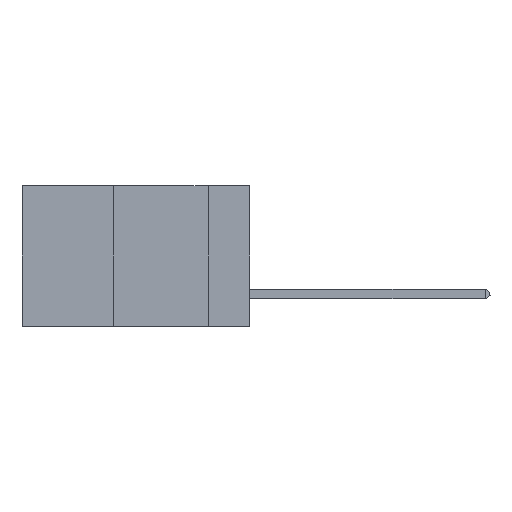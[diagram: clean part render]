
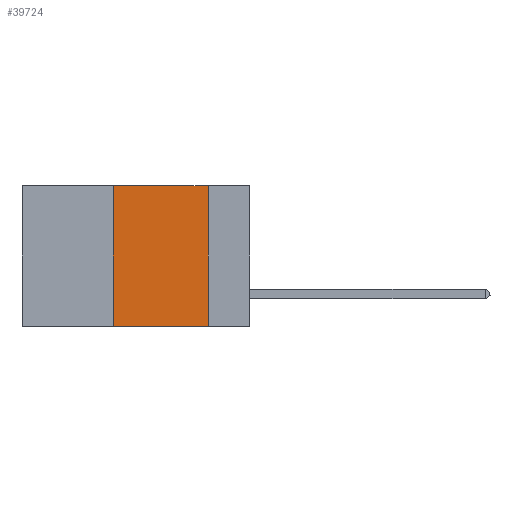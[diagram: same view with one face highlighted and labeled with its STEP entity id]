
A CAD part, left-side view. The second image highlights one B-rep face of the part: STEP entity #39724.
In plain terms, the highlighted planar face has unit normal (-1, 0, 0).
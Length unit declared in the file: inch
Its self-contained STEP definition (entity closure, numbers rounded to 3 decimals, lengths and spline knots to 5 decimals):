
#577 = FACE_OUTER_BOUND ( 'NONE', #27280, .T. ) ;
#1694 = DIRECTION ( 'NONE',  ( 0., 0., 1. ) ) ;
#2815 = VERTEX_POINT ( 'NONE', #20544 ) ;
#5615 = CARTESIAN_POINT ( 'NONE',  ( 0., 0.36, 0. ) ) ;
#7092 = CARTESIAN_POINT ( 'NONE',  ( 0., 0.11, 0. ) ) ;
#7485 = VECTOR ( 'NONE', #1694, 39.37008 ) ;
#9587 = ORIENTED_EDGE ( 'NONE', *, *, #45591, .F. ) ;
#9704 = DIRECTION ( 'NONE',  ( 0., -1., 0. ) ) ;
#9716 = VECTOR ( 'NONE', #43113, 39.37008 ) ;
#10158 = AXIS2_PLACEMENT_3D ( 'NONE', #39242, #46768, #35796 ) ;
#10191 = CARTESIAN_POINT ( 'NONE',  ( 0., 0.36, -0.37 ) ) ;
#10508 = VECTOR ( 'NONE', #29801, 39.37008 ) ;
#10557 = VERTEX_POINT ( 'NONE', #10191 ) ;
#14171 = ORIENTED_EDGE ( 'NONE', *, *, #23688, .T. ) ;
#16242 = VERTEX_POINT ( 'NONE', #26214 ) ;
#17302 = EDGE_CURVE ( 'NONE', #16242, #23471, #37473, .T. ) ;
#20544 = CARTESIAN_POINT ( 'NONE',  ( 0., 0.36, 0. ) ) ;
#20882 = PLANE ( 'NONE',  #10158 ) ;
#21519 = LINE ( 'NONE', #5615, #7485 ) ;
#22015 = LINE ( 'NONE', #35717, #34338 ) ;
#23471 = VERTEX_POINT ( 'NONE', #38985 ) ;
#23688 = EDGE_CURVE ( 'NONE', #10557, #23471, #22015, .T. ) ;
#26214 = CARTESIAN_POINT ( 'NONE',  ( 0., 0.11, 0. ) ) ;
#27280 = EDGE_LOOP ( 'NONE', ( #32638, #46162, #9587, #14171 ) ) ;
#29801 = DIRECTION ( 'NONE',  ( 0., 0., -1. ) ) ;
#31628 = CARTESIAN_POINT ( 'NONE',  ( 0., 0.6, 0. ) ) ;
#32638 = ORIENTED_EDGE ( 'NONE', *, *, #17302, .F. ) ;
#34338 = VECTOR ( 'NONE', #9704, 39.37008 ) ;
#34866 = LINE ( 'NONE', #31628, #9716 ) ;
#35717 = CARTESIAN_POINT ( 'NONE',  ( 0., 0.6, -0.37 ) ) ;
#35796 = DIRECTION ( 'NONE',  ( 0., 0., -1. ) ) ;
#37473 = LINE ( 'NONE', #7092, #10508 ) ;
#38985 = CARTESIAN_POINT ( 'NONE',  ( 0., 0.11, -0.37 ) ) ;
#39242 = CARTESIAN_POINT ( 'NONE',  ( 0., 0.6, 0. ) ) ;
#39724 = ADVANCED_FACE ( 'NONE', ( #577 ), #20882, .F. ) ;
#43113 = DIRECTION ( 'NONE',  ( 0., -1., 0. ) ) ;
#45591 = EDGE_CURVE ( 'NONE', #10557, #2815, #21519, .T. ) ;
#46162 = ORIENTED_EDGE ( 'NONE', *, *, #47052, .F. ) ;
#46768 = DIRECTION ( 'NONE',  ( 1., 0., 0. ) ) ;
#47052 = EDGE_CURVE ( 'NONE', #2815, #16242, #34866, .T. ) ;
